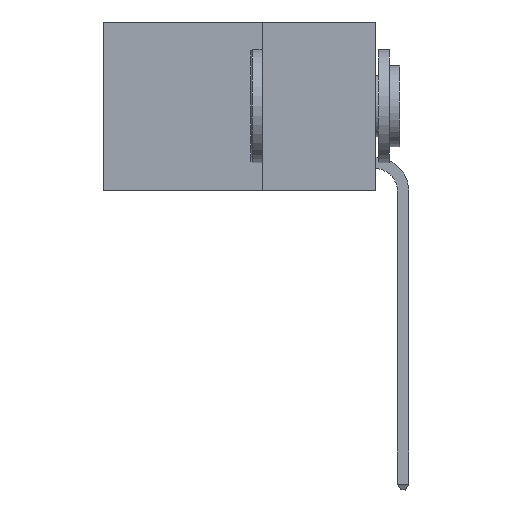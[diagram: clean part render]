
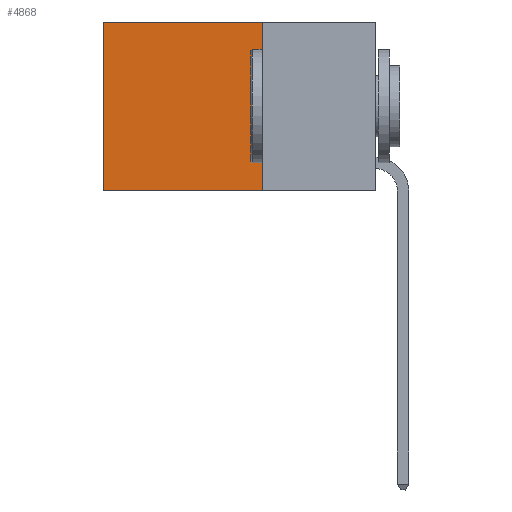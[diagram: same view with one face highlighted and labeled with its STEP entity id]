
A CAD part, left-side view. The second image highlights one B-rep face of the part: STEP entity #4868.
In plain terms, the highlighted planar face has unit normal (-1, 0, 0).
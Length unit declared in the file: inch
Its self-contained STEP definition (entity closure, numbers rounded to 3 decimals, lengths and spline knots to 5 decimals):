
#880 = VECTOR ( 'NONE', #5179, 39.37008 ) ;
#1503 = VECTOR ( 'NONE', #11153, 39.37008 ) ;
#1960 = CARTESIAN_POINT ( 'NONE',  ( 0.2625, 0.25, -0.37 ) ) ;
#2160 = DIRECTION ( 'NONE',  ( 0., 0., -1. ) ) ;
#2981 = CARTESIAN_POINT ( 'NONE',  ( 0.2625, 0.6, 0. ) ) ;
#3337 = LINE ( 'NONE', #8794, #880 ) ;
#4598 = VERTEX_POINT ( 'NONE', #10497 ) ;
#4779 = DIRECTION ( 'NONE',  ( 0., 0., -1. ) ) ;
#4868 = ADVANCED_FACE ( 'NONE', ( #7288 ), #8475, .F. ) ;
#5133 = ORIENTED_EDGE ( 'NONE', *, *, #7237, .T. ) ;
#5177 = ORIENTED_EDGE ( 'NONE', *, *, #7610, .F. ) ;
#5178 = ORIENTED_EDGE ( 'NONE', *, *, #5916, .F. ) ;
#5179 = DIRECTION ( 'NONE',  ( 0., 0., -1. ) ) ;
#5252 = ORIENTED_EDGE ( 'NONE', *, *, #5710, .T. ) ;
#5420 = VERTEX_POINT ( 'NONE', #10327 ) ;
#5703 = CARTESIAN_POINT ( 'NONE',  ( 0.2625, 0.25, 0. ) ) ;
#5710 = EDGE_CURVE ( 'NONE', #5420, #8082, #9216, .T. ) ;
#5852 = VECTOR ( 'NONE', #2160, 39.37008 ) ;
#5916 = EDGE_CURVE ( 'NONE', #5420, #9753, #8295, .T. ) ;
#5928 = CARTESIAN_POINT ( 'NONE',  ( 0.2625, 0.25, 0. ) ) ;
#6438 = LINE ( 'NONE', #10289, #1503 ) ;
#7237 = EDGE_CURVE ( 'NONE', #8082, #4598, #3337, .T. ) ;
#7288 = FACE_OUTER_BOUND ( 'NONE', #9054, .T. ) ;
#7610 = EDGE_CURVE ( 'NONE', #9753, #4598, #6438, .T. ) ;
#8082 = VERTEX_POINT ( 'NONE', #2981 ) ;
#8295 = LINE ( 'NONE', #5928, #5852 ) ;
#8475 = PLANE ( 'NONE',  #10402 ) ;
#8794 = CARTESIAN_POINT ( 'NONE',  ( 0.2625, 0.6, 0. ) ) ;
#9054 = EDGE_LOOP ( 'NONE', ( #5133, #5177, #5178, #5252 ) ) ;
#9216 = LINE ( 'NONE', #10859, #9485 ) ;
#9485 = VECTOR ( 'NONE', #11689, 39.37008 ) ;
#9753 = VERTEX_POINT ( 'NONE', #1960 ) ;
#10152 = DIRECTION ( 'NONE',  ( 1., 0., 0. ) ) ;
#10289 = CARTESIAN_POINT ( 'NONE',  ( 0.2625, 0.25, -0.37 ) ) ;
#10327 = CARTESIAN_POINT ( 'NONE',  ( 0.2625, 0.25, 0. ) ) ;
#10402 = AXIS2_PLACEMENT_3D ( 'NONE', #5703, #10152, #4779 ) ;
#10497 = CARTESIAN_POINT ( 'NONE',  ( 0.2625, 0.6, -0.37 ) ) ;
#10859 = CARTESIAN_POINT ( 'NONE',  ( 0.2625, 0.25, 0. ) ) ;
#11153 = DIRECTION ( 'NONE',  ( 0., 1., 0. ) ) ;
#11689 = DIRECTION ( 'NONE',  ( 0., 1., 0. ) ) ;
